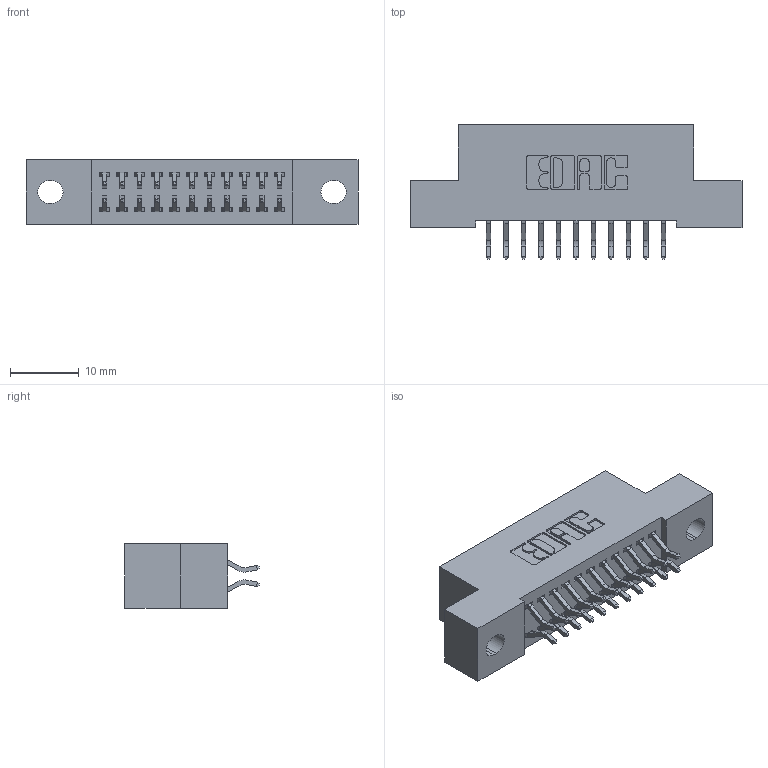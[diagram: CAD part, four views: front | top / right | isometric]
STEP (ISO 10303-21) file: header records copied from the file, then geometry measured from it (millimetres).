
FILE_DESCRIPTION (( 'STEP AP203' ), '1' );
FILE_NAME ('342-022-556-202.STEP', '2018-08-11T00:58:49', ( '' ), ( '' ), 'SwSTEP 2.0', 'SolidWorks 2016', '' );
FILE_SCHEMA (( 'CONFIG_CONTROL_DESIGN' ));
Length unit declared in the file: inch
Products named in the file (3): 345-292-001_556 Tail; 342-022-556-202; 342 Part_.128 Slot
Assembly tree (23 placements, depth 2):
  342-022-556-202
    342 Part_.128 Slot
    345-292-001_556 Tail  x22
Bounding box: 48.26 x 19.58 x 9.4 mm (x, y, z)
Volume: 4136.7 mm3; surface area: 5707.8 mm2
Topology: 23 solids, 23 shells, 1390 faces, 4117 edges, 2714 vertices
Faces by surface type: plane 950, cylinder 440
Entity records: 11309 total; most frequent: CARTESIAN_POINT 1926, ORIENTED_EDGE 1850, DIRECTION 1689, EDGE_CURVE 925, VECTOR 789, LINE 789, VERTEX_POINT 614, AXIS2_PLACEMENT_3D 450
